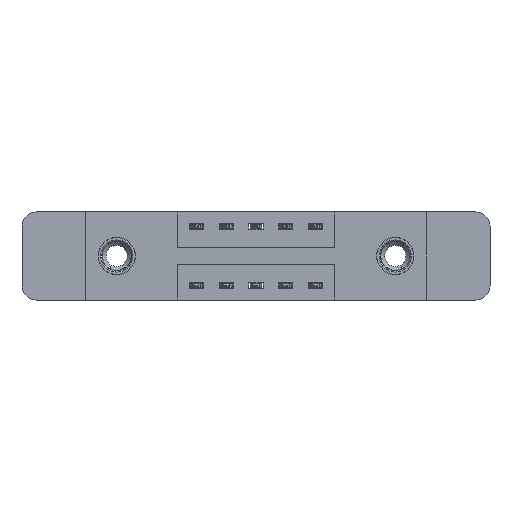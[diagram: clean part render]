
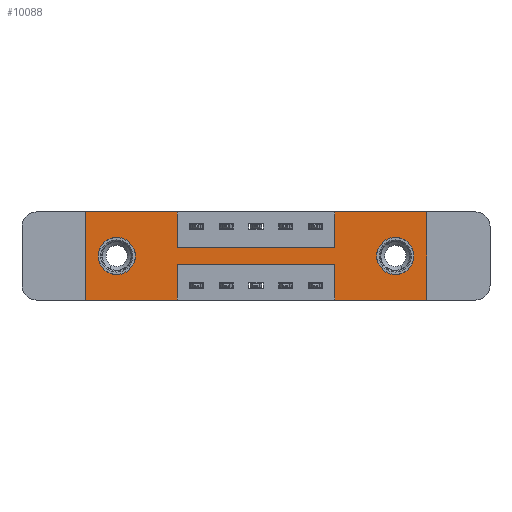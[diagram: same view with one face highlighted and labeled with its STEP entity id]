
A CAD part, front view. The second image highlights one B-rep face of the part: STEP entity #10088.
In plain terms, the highlighted planar face has unit normal (0, -1, 0).
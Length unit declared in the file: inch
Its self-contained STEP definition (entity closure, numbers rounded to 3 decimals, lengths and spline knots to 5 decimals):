
#188 = VERTEX_POINT ( 'NONE', #5538 ) ;
#313 = DIRECTION ( 'NONE',  ( 0., 1., 0. ) ) ;
#474 = CARTESIAN_POINT ( 'NONE',  ( 1.0475, 0., 0. ) ) ;
#475 = FACE_BOUND ( 'NONE', #4416, .T. ) ;
#979 = DIRECTION ( 'NONE',  ( 0., 0., -1. ) ) ;
#1144 = EDGE_CURVE ( 'NONE', #10795, #1776, #5005, .T. ) ;
#1274 = VERTEX_POINT ( 'NONE', #4099 ) ;
#1443 = CARTESIAN_POINT ( 'NONE',  ( 0., 0., -0.37 ) ) ;
#1449 = ORIENTED_EDGE ( 'NONE', *, *, #1144, .F. ) ;
#1472 = CARTESIAN_POINT ( 'NONE',  ( 0., 0., -0.37 ) ) ;
#1484 = VERTEX_POINT ( 'NONE', #11477 ) ;
#1499 = EDGE_LOOP ( 'NONE', ( #12111, #8349, #1897, #6054, #9846, #9794, #9000, #13181, #1449, #11032, #5332, #11123 ) ) ;
#1703 = VERTEX_POINT ( 'NONE', #6471 ) ;
#1776 = VERTEX_POINT ( 'NONE', #2632 ) ;
#1897 = ORIENTED_EDGE ( 'NONE', *, *, #13316, .F. ) ;
#1970 = CARTESIAN_POINT ( 'NONE',  ( 0.1325, 0., -0.107 ) ) ;
#1989 = VERTEX_POINT ( 'NONE', #2774 ) ;
#2005 = CIRCLE ( 'NONE', #2911, 0.078 ) ;
#2220 = EDGE_CURVE ( 'NONE', #11981, #10795, #4590, .T. ) ;
#2369 = DIRECTION ( 'NONE',  ( -1., 0., 0. ) ) ;
#2381 = EDGE_CURVE ( 'NONE', #188, #4287, #3951, .T. ) ;
#2482 = EDGE_CURVE ( 'NONE', #13082, #11981, #5870, .T. ) ;
#2510 = LINE ( 'NONE', #4425, #10371 ) ;
#2617 = CARTESIAN_POINT ( 'NONE',  ( 1.0475, 0., -0.37 ) ) ;
#2632 = CARTESIAN_POINT ( 'NONE',  ( 0.3875, 0., -0.15 ) ) ;
#2770 = VERTEX_POINT ( 'NONE', #3331 ) ;
#2774 = CARTESIAN_POINT ( 'NONE',  ( 0.3875, 0., -0.37 ) ) ;
#2903 = CARTESIAN_POINT ( 'NONE',  ( 0.3875, 0., -0.22 ) ) ;
#2911 = AXIS2_PLACEMENT_3D ( 'NONE', #3586, #6782, #13479 ) ;
#3040 = LINE ( 'NONE', #11513, #13512 ) ;
#3093 = EDGE_CURVE ( 'NONE', #6070, #2770, #13481, .T. ) ;
#3331 = CARTESIAN_POINT ( 'NONE',  ( 0.1325, 0., -0.263 ) ) ;
#3523 = ORIENTED_EDGE ( 'NONE', *, *, #4739, .T. ) ;
#3574 = DIRECTION ( 'NONE',  ( 0., 0., 1. ) ) ;
#3586 = CARTESIAN_POINT ( 'NONE',  ( 0.1325, 0., -0.185 ) ) ;
#3669 = DIRECTION ( 'NONE',  ( -1., 0., 0. ) ) ;
#3675 = EDGE_CURVE ( 'NONE', #1484, #11822, #13228, .T. ) ;
#3806 = CIRCLE ( 'NONE', #12168, 0.078 ) ;
#3951 = LINE ( 'NONE', #2903, #11654 ) ;
#3967 = AXIS2_PLACEMENT_3D ( 'NONE', #12237, #9057, #13372 ) ;
#4021 = DIRECTION ( 'NONE',  ( 0., 0., 1. ) ) ;
#4099 = CARTESIAN_POINT ( 'NONE',  ( 1.0475, 0., -0.15 ) ) ;
#4162 = VECTOR ( 'NONE', #9053, 39.37008 ) ;
#4171 = CARTESIAN_POINT ( 'NONE',  ( 1.3025, 0., -0.185 ) ) ;
#4287 = VERTEX_POINT ( 'NONE', #11633 ) ;
#4321 = CARTESIAN_POINT ( 'NONE',  ( 0., 0., 0. ) ) ;
#4416 = EDGE_LOOP ( 'NONE', ( #8239, #9058 ) ) ;
#4425 = CARTESIAN_POINT ( 'NONE',  ( 0., 0., 0. ) ) ;
#4532 = CARTESIAN_POINT ( 'NONE',  ( 0., 0., 0. ) ) ;
#4552 = VERTEX_POINT ( 'NONE', #2617 ) ;
#4590 = LINE ( 'NONE', #4532, #4630 ) ;
#4630 = VECTOR ( 'NONE', #13094, 39.37008 ) ;
#4677 = CARTESIAN_POINT ( 'NONE',  ( 0.3875, 0., -0.15 ) ) ;
#4739 = EDGE_CURVE ( 'NONE', #11822, #1484, #3806, .T. ) ;
#4792 = DIRECTION ( 'NONE',  ( -1., 0., 0. ) ) ;
#4894 = CARTESIAN_POINT ( 'NONE',  ( 1.3025, 0., -0.107 ) ) ;
#4978 = LINE ( 'NONE', #5907, #11832 ) ;
#5005 = LINE ( 'NONE', #10168, #4162 ) ;
#5298 = DIRECTION ( 'NONE',  ( 0., 0., 1. ) ) ;
#5332 = ORIENTED_EDGE ( 'NONE', *, *, #2482, .F. ) ;
#5538 = CARTESIAN_POINT ( 'NONE',  ( 1.0475, 0., -0.22 ) ) ;
#5668 = EDGE_CURVE ( 'NONE', #1776, #1274, #9980, .T. ) ;
#5762 = VECTOR ( 'NONE', #4792, 39.37008 ) ;
#5785 = DIRECTION ( 'NONE',  ( 0., -1., 0. ) ) ;
#5852 = AXIS2_PLACEMENT_3D ( 'NONE', #1472, #5785, #9960 ) ;
#5870 = LINE ( 'NONE', #4321, #13476 ) ;
#5907 = CARTESIAN_POINT ( 'NONE',  ( 0.3875, 0., -0.37 ) ) ;
#5932 = CARTESIAN_POINT ( 'NONE',  ( 0., 0., -0.37 ) ) ;
#5962 = DIRECTION ( 'NONE',  ( 0., 0., -1. ) ) ;
#6054 = ORIENTED_EDGE ( 'NONE', *, *, #11196, .F. ) ;
#6070 = VERTEX_POINT ( 'NONE', #1970 ) ;
#6143 = CARTESIAN_POINT ( 'NONE',  ( 0., 0., 0. ) ) ;
#6277 = EDGE_CURVE ( 'NONE', #4287, #1989, #4978, .T. ) ;
#6344 = CARTESIAN_POINT ( 'NONE',  ( 1.435, 0., 0. ) ) ;
#6471 = CARTESIAN_POINT ( 'NONE',  ( 1.435, 0., -0.37 ) ) ;
#6768 = CARTESIAN_POINT ( 'NONE',  ( 0.1325, 0., -0.185 ) ) ;
#6782 = DIRECTION ( 'NONE',  ( 0., 1., 0. ) ) ;
#6997 = LINE ( 'NONE', #5932, #5762 ) ;
#7047 = CARTESIAN_POINT ( 'NONE',  ( 1.0475, 0., -0.37 ) ) ;
#7097 = CARTESIAN_POINT ( 'NONE',  ( 1.435, 0., 0. ) ) ;
#7310 = VECTOR ( 'NONE', #9209, 39.37008 ) ;
#7945 = LINE ( 'NONE', #7097, #13650 ) ;
#8066 = EDGE_CURVE ( 'NONE', #12589, #1703, #7945, .T. ) ;
#8123 = CARTESIAN_POINT ( 'NONE',  ( 0., 0., -0.37 ) ) ;
#8239 = ORIENTED_EDGE ( 'NONE', *, *, #3093, .T. ) ;
#8349 = ORIENTED_EDGE ( 'NONE', *, *, #2381, .F. ) ;
#9000 = ORIENTED_EDGE ( 'NONE', *, *, #11406, .F. ) ;
#9053 = DIRECTION ( 'NONE',  ( 0., 0., -1. ) ) ;
#9057 = DIRECTION ( 'NONE',  ( 0., 1., 0. ) ) ;
#9058 = ORIENTED_EDGE ( 'NONE', *, *, #11628, .T. ) ;
#9103 = EDGE_CURVE ( 'NONE', #11945, #12589, #2510, .T. ) ;
#9209 = DIRECTION ( 'NONE',  ( 1., 0., 0. ) ) ;
#9794 = ORIENTED_EDGE ( 'NONE', *, *, #9103, .F. ) ;
#9846 = ORIENTED_EDGE ( 'NONE', *, *, #8066, .F. ) ;
#9922 = VECTOR ( 'NONE', #13410, 39.37008 ) ;
#9960 = DIRECTION ( 'NONE',  ( 0., 0., -1. ) ) ;
#9980 = LINE ( 'NONE', #4677, #7310 ) ;
#10028 = PLANE ( 'NONE',  #5852 ) ;
#10088 = ADVANCED_FACE ( 'NONE', ( #10163, #475, #13433 ), #10028, .T. ) ;
#10163 = FACE_BOUND ( 'NONE', #10660, .T. ) ;
#10168 = CARTESIAN_POINT ( 'NONE',  ( 0.3875, 0., 0. ) ) ;
#10371 = VECTOR ( 'NONE', #11125, 39.37008 ) ;
#10645 = CARTESIAN_POINT ( 'NONE',  ( 0.3875, 0., 0. ) ) ;
#10660 = EDGE_LOOP ( 'NONE', ( #3523, #11652 ) ) ;
#10795 = VERTEX_POINT ( 'NONE', #10645 ) ;
#10857 = EDGE_CURVE ( 'NONE', #1989, #13082, #12055, .T. ) ;
#11032 = ORIENTED_EDGE ( 'NONE', *, *, #2220, .F. ) ;
#11123 = ORIENTED_EDGE ( 'NONE', *, *, #10857, .F. ) ;
#11125 = DIRECTION ( 'NONE',  ( 1., 0., 0. ) ) ;
#11196 = EDGE_CURVE ( 'NONE', #1703, #4552, #6997, .T. ) ;
#11406 = EDGE_CURVE ( 'NONE', #1274, #11945, #3040, .T. ) ;
#11414 = DIRECTION ( 'NONE',  ( 0., 0., -1. ) ) ;
#11477 = CARTESIAN_POINT ( 'NONE',  ( 1.3025, 0., -0.263 ) ) ;
#11513 = CARTESIAN_POINT ( 'NONE',  ( 1.0475, 0., 0. ) ) ;
#11628 = EDGE_CURVE ( 'NONE', #2770, #6070, #2005, .T. ) ;
#11633 = CARTESIAN_POINT ( 'NONE',  ( 0.3875, 0., -0.22 ) ) ;
#11652 = ORIENTED_EDGE ( 'NONE', *, *, #3675, .T. ) ;
#11654 = VECTOR ( 'NONE', #3669, 39.37008 ) ;
#11822 = VERTEX_POINT ( 'NONE', #4894 ) ;
#11832 = VECTOR ( 'NONE', #11414, 39.37008 ) ;
#11945 = VERTEX_POINT ( 'NONE', #474 ) ;
#11981 = VERTEX_POINT ( 'NONE', #6143 ) ;
#12055 = LINE ( 'NONE', #1443, #12801 ) ;
#12111 = ORIENTED_EDGE ( 'NONE', *, *, #6277, .F. ) ;
#12168 = AXIS2_PLACEMENT_3D ( 'NONE', #4171, #12660, #979 ) ;
#12237 = CARTESIAN_POINT ( 'NONE',  ( 1.3025, 0., -0.185 ) ) ;
#12589 = VERTEX_POINT ( 'NONE', #6344 ) ;
#12660 = DIRECTION ( 'NONE',  ( 0., 1., 0. ) ) ;
#12801 = VECTOR ( 'NONE', #2369, 39.37008 ) ;
#12825 = AXIS2_PLACEMENT_3D ( 'NONE', #6768, #313, #3574 ) ;
#13082 = VERTEX_POINT ( 'NONE', #8123 ) ;
#13094 = DIRECTION ( 'NONE',  ( 1., 0., 0. ) ) ;
#13181 = ORIENTED_EDGE ( 'NONE', *, *, #5668, .F. ) ;
#13228 = CIRCLE ( 'NONE', #3967, 0.078 ) ;
#13316 = EDGE_CURVE ( 'NONE', #4552, #188, #13478, .T. ) ;
#13372 = DIRECTION ( 'NONE',  ( 0., 0., -1. ) ) ;
#13410 = DIRECTION ( 'NONE',  ( 0., 0., 1. ) ) ;
#13433 = FACE_OUTER_BOUND ( 'NONE', #1499, .T. ) ;
#13476 = VECTOR ( 'NONE', #5298, 39.37008 ) ;
#13478 = LINE ( 'NONE', #7047, #9922 ) ;
#13479 = DIRECTION ( 'NONE',  ( 0., 0., 1. ) ) ;
#13481 = CIRCLE ( 'NONE', #12825, 0.078 ) ;
#13512 = VECTOR ( 'NONE', #4021, 39.37008 ) ;
#13650 = VECTOR ( 'NONE', #5962, 39.37008 ) ;
